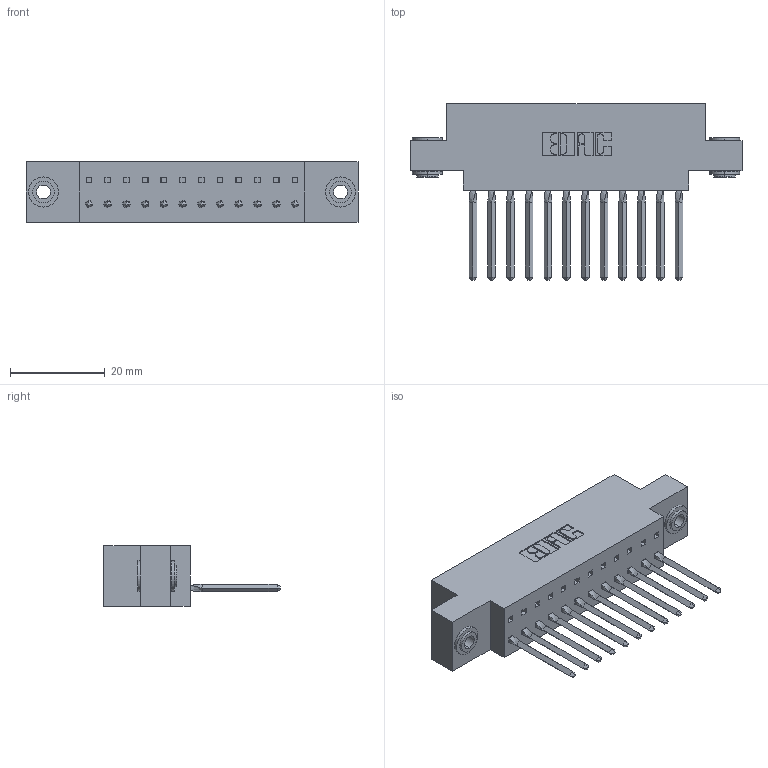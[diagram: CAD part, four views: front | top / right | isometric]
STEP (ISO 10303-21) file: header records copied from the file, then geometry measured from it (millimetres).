
FILE_DESCRIPTION (( 'STEP AP203' ), '1' );
FILE_NAME ('317-012-541-603.STEP', '2020-02-27T13:58:31', ( '' ), ( '' ), 'SwSTEP 2.0', 'SolidWorks 2016', '' );
FILE_SCHEMA (( 'CONFIG_CONTROL_DESIGN' ));
Length unit declared in the file: inch
Products named in the file (4): 317-012-541-603; 345-250-002_345-250-002-102; 317 Part_.156 Dia - TH; 317-290-002_541
Assembly tree (15 placements, depth 2):
  317-012-541-603
    317 Part_.156 Dia - TH
    317-290-002_541  x12
    345-250-002_345-250-002-102  x2
Bounding box: 70.26 x 37.34 x 12.7 mm (x, y, z)
Volume: 10490.2 mm3; surface area: 14037.8 mm2
Topology: 15 solids, 15 shells, 1964 faces, 5559 edges, 3614 vertices
Faces by surface type: plane 1556, cylinder 352, bspline 48, cone 8
Entity records: 23345 total; most frequent: CARTESIAN_POINT 4744, ORIENTED_EDGE 4002, DIRECTION 3307, EDGE_CURVE 2001, VECTOR 1613, LINE 1613, VERTEX_POINT 1324, AXIS2_PLACEMENT_3D 847
